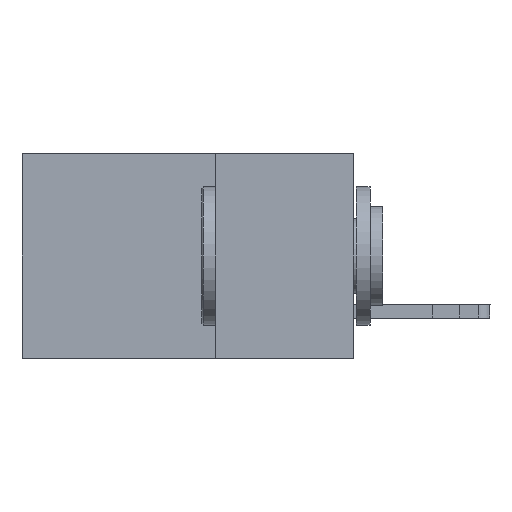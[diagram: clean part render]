
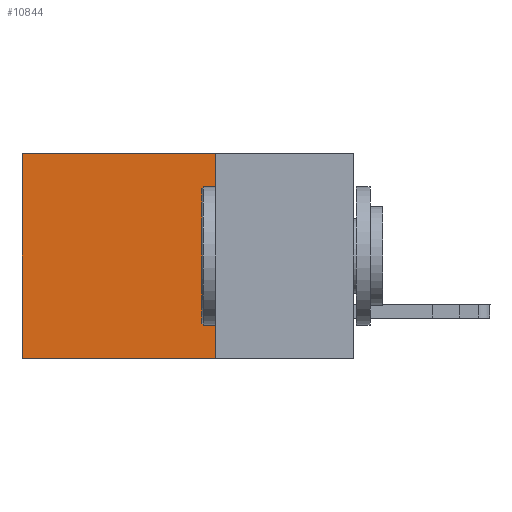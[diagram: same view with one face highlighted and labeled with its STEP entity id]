
A CAD part, left-side view. The second image highlights one B-rep face of the part: STEP entity #10844.
In plain terms, the highlighted planar face has unit normal (-1, 0, 0).
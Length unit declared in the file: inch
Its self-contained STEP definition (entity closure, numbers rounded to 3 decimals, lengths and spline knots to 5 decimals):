
#128 = EDGE_LOOP ( 'NONE', ( #4027, #5881, #11739, #12438 ) ) ;
#341 = EDGE_CURVE ( 'NONE', #5323, #6242, #12010, .T. ) ;
#1640 = EDGE_CURVE ( 'NONE', #9149, #11017, #11571, .T. ) ;
#1696 = CARTESIAN_POINT ( 'NONE',  ( 0.2875, 0.25, 0. ) ) ;
#2180 = CARTESIAN_POINT ( 'NONE',  ( 0.2875, 0.25, 0. ) ) ;
#2227 = DIRECTION ( 'NONE',  ( 0., 1., 0. ) ) ;
#2482 = CARTESIAN_POINT ( 'NONE',  ( 0.2875, 0.6, -0.37 ) ) ;
#3037 = CARTESIAN_POINT ( 'NONE',  ( 0.2875, 0.25, 0. ) ) ;
#4027 = ORIENTED_EDGE ( 'NONE', *, *, #15902, .T. ) ;
#5323 = VERTEX_POINT ( 'NONE', #3037 ) ;
#5881 = ORIENTED_EDGE ( 'NONE', *, *, #1640, .F. ) ;
#6076 = AXIS2_PLACEMENT_3D ( 'NONE', #9467, #15862, #7048 ) ;
#6242 = VERTEX_POINT ( 'NONE', #14152 ) ;
#6492 = EDGE_CURVE ( 'NONE', #5323, #9149, #15898, .T. ) ;
#6980 = CARTESIAN_POINT ( 'NONE',  ( 0.2875, 0.25, -0.37 ) ) ;
#7048 = DIRECTION ( 'NONE',  ( 0., 0., -1. ) ) ;
#9149 = VERTEX_POINT ( 'NONE', #10525 ) ;
#9467 = CARTESIAN_POINT ( 'NONE',  ( 0.2875, 0.25, 0. ) ) ;
#10346 = CARTESIAN_POINT ( 'NONE',  ( 0.2875, 0.6, 0. ) ) ;
#10525 = CARTESIAN_POINT ( 'NONE',  ( 0.2875, 0.25, -0.37 ) ) ;
#10844 = ADVANCED_FACE ( 'NONE', ( #15601 ), #14514, .F. ) ;
#10929 = DIRECTION ( 'NONE',  ( 0., 0., -1. ) ) ;
#11017 = VERTEX_POINT ( 'NONE', #2482 ) ;
#11571 = LINE ( 'NONE', #6980, #12543 ) ;
#11739 = ORIENTED_EDGE ( 'NONE', *, *, #6492, .F. ) ;
#12010 = LINE ( 'NONE', #1696, #14538 ) ;
#12438 = ORIENTED_EDGE ( 'NONE', *, *, #341, .T. ) ;
#12543 = VECTOR ( 'NONE', #2227, 39.37008 ) ;
#12593 = VECTOR ( 'NONE', #10929, 39.37008 ) ;
#13631 = VECTOR ( 'NONE', #14324, 39.37008 ) ;
#14152 = CARTESIAN_POINT ( 'NONE',  ( 0.2875, 0.6, 0. ) ) ;
#14324 = DIRECTION ( 'NONE',  ( 0., 0., -1. ) ) ;
#14514 = PLANE ( 'NONE',  #6076 ) ;
#14538 = VECTOR ( 'NONE', #15429, 39.37008 ) ;
#15429 = DIRECTION ( 'NONE',  ( 0., 1., 0. ) ) ;
#15601 = FACE_OUTER_BOUND ( 'NONE', #128, .T. ) ;
#15862 = DIRECTION ( 'NONE',  ( 1., 0., 0. ) ) ;
#15898 = LINE ( 'NONE', #2180, #12593 ) ;
#15902 = EDGE_CURVE ( 'NONE', #6242, #11017, #16142, .T. ) ;
#16142 = LINE ( 'NONE', #10346, #13631 ) ;
